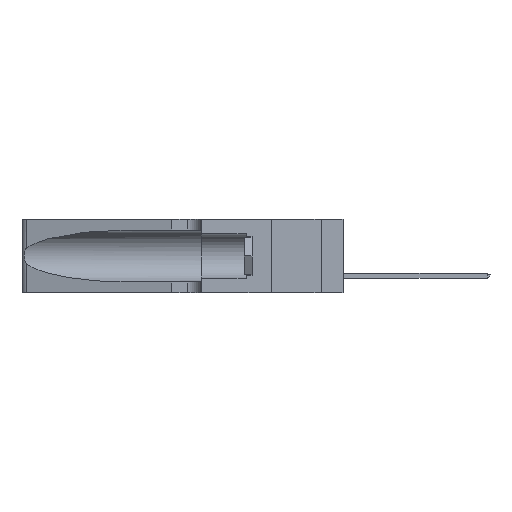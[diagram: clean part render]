
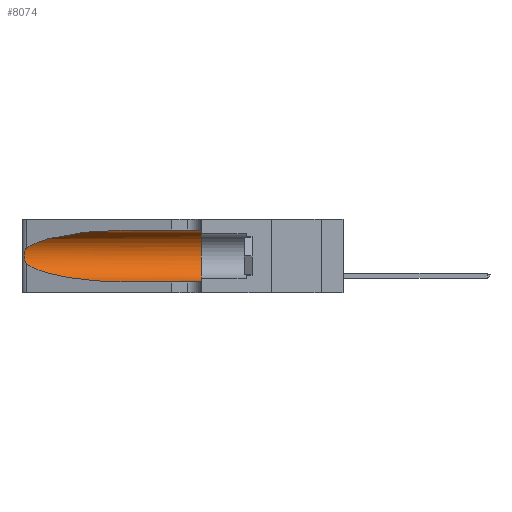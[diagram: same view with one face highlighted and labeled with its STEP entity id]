
A CAD part, left-side view. The second image highlights one B-rep face of the part: STEP entity #8074.
In plain terms, the highlighted cylindrical face has radius 3.308 mm (diameter 6.617 mm), a partial arc.
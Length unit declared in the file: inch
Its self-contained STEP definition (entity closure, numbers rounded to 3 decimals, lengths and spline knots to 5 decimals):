
#131 = EDGE_CURVE ( 'NONE', #30918, #43896, #28173, .T. ) ;
#206 = AXIS2_PLACEMENT_3D ( 'NONE', #17115, #22772, #15755 ) ;
#1031 = CARTESIAN_POINT ( 'NONE',  ( 0.1305, 0.35, 0.05475 ) ) ;
#1728 = B_SPLINE_CURVE_WITH_KNOTS ( 'NONE', 3,
 ( #28194, #2539, #35763, #24893, #32427, #6935, #26550, #5918, #18205, #4153, #21812, #35716, #33601, #24954 ),
 .UNSPECIFIED., .F., .F.,
 ( 4, 2, 2, 2, 2, 2, 4 ),
 ( 0., 0.00027, 0.00053, 0.00107, 0.0016, 0.00187, 0.00214 ),
 .UNSPECIFIED. ) ;
#2324 = DIRECTION ( 'NONE',  ( 0., 0., -1. ) ) ;
#2539 = CARTESIAN_POINT ( 'NONE',  ( 0.25555, 1.22994, 0.2215 ) ) ;
#4153 = CARTESIAN_POINT ( 'NONE',  ( 0.25856, 1.23593, 0.16098 ) ) ;
#4603 = CARTESIAN_POINT ( 'NONE',  ( 0.25487, 1.22718, 0.22369 ) ) ;
#4626 =( BOUNDED_CURVE ( )  B_SPLINE_CURVE ( 3, ( #16541, #5074, #40308, #4603 ),
 .UNSPECIFIED., .F., .F. ) 
 B_SPLINE_CURVE_WITH_KNOTS ( ( 4, 4 ),
 ( 1.5708, 2.84003 ),
 .UNSPECIFIED. ) 
 CURVE ( )  GEOMETRIC_REPRESENTATION_ITEM ( )  RATIONAL_B_SPLINE_CURVE ( ( 1., 0.87, 0.87, 1. ) ) 
 REPRESENTATION_ITEM ( '' )  );
#4814 = DIRECTION ( 'NONE',  ( 0., -1., 0. ) ) ;
#4993 = CARTESIAN_POINT ( 'NONE',  ( 0.1305, 1.61858, 0.185 ) ) ;
#5074 = CARTESIAN_POINT ( 'NONE',  ( 0.18966, 0.96281, 0.31525 ) ) ;
#5448 = VERTEX_POINT ( 'NONE', #12905 ) ;
#5918 = CARTESIAN_POINT ( 'NONE',  ( 0.26075, 1.23896, 0.178 ) ) ;
#6399 = AXIS2_PLACEMENT_3D ( 'NONE', #4993, #19834, #2324 ) ;
#6935 = CARTESIAN_POINT ( 'NONE',  ( 0.26018, 1.23835, 0.19895 ) ) ;
#7146 = VERTEX_POINT ( 'NONE', #20225 ) ;
#7177 = CARTESIAN_POINT ( 'NONE',  ( 0.1305, 0.72297, 0.05475 ) ) ;
#7423 = CARTESIAN_POINT ( 'NONE',  ( 0.1305, 0.72297, 0.05475 ) ) ;
#8074 = ADVANCED_FACE ( 'NONE', ( #23088 ), #19157, .F. ) ;
#8538 = ORIENTED_EDGE ( 'NONE', *, *, #16496, .T. ) ;
#8761 = CARTESIAN_POINT ( 'NONE',  ( 0.1305, 1.61858, 0.05475 ) ) ;
#9123 = ORIENTED_EDGE ( 'NONE', *, *, #36473, .F. ) ;
#9232 = LINE ( 'NONE', #22787, #46150 ) ;
#11258 = EDGE_CURVE ( 'NONE', #43896, #36379, #15746, .T. ) ;
#12360 = EDGE_CURVE ( 'NONE', #5448, #30918, #1728, .T. ) ;
#12905 = CARTESIAN_POINT ( 'NONE',  ( 0.25487, 1.22718, 0.22369 ) ) ;
#13429 = EDGE_CURVE ( 'NONE', #15720, #36379, #40744, .T. ) ;
#15720 = VERTEX_POINT ( 'NONE', #25858 ) ;
#15746 = LINE ( 'NONE', #8761, #39845 ) ;
#15755 = DIRECTION ( 'NONE',  ( 0., 0., 1. ) ) ;
#16496 = EDGE_CURVE ( 'NONE', #7146, #5448, #4626, .T. ) ;
#16541 = CARTESIAN_POINT ( 'NONE',  ( 0.1305, 0.72297, 0.31525 ) ) ;
#17115 = CARTESIAN_POINT ( 'NONE',  ( 0.1305, 0.35, 0.185 ) ) ;
#18205 = CARTESIAN_POINT ( 'NONE',  ( 0.26017, 1.23833, 0.17102 ) ) ;
#19157 = CYLINDRICAL_SURFACE ( 'NONE', #6399, 0.13025 ) ;
#19531 = ORIENTED_EDGE ( 'NONE', *, *, #11258, .T. ) ;
#19834 = DIRECTION ( 'NONE',  ( 0., -1., 0. ) ) ;
#20225 = CARTESIAN_POINT ( 'NONE',  ( 0.1305, 0.72297, 0.31525 ) ) ;
#21625 = CARTESIAN_POINT ( 'NONE',  ( 0.2373, 1.15595, 0.08982 ) ) ;
#21812 = CARTESIAN_POINT ( 'NONE',  ( 0.25789, 1.23486, 0.15765 ) ) ;
#22772 = DIRECTION ( 'NONE',  ( 0., 1., 0. ) ) ;
#22787 = CARTESIAN_POINT ( 'NONE',  ( 0.1305, 1.61858, 0.31525 ) ) ;
#23088 = FACE_OUTER_BOUND ( 'NONE', #45938, .T. ) ;
#24893 = CARTESIAN_POINT ( 'NONE',  ( 0.25787, 1.23484, 0.2124 ) ) ;
#24954 = CARTESIAN_POINT ( 'NONE',  ( 0.25487, 1.22718, 0.14631 ) ) ;
#25858 = CARTESIAN_POINT ( 'NONE',  ( 0.1305, 0.35, 0.31525 ) ) ;
#26370 = ORIENTED_EDGE ( 'NONE', *, *, #12360, .T. ) ;
#26550 = CARTESIAN_POINT ( 'NONE',  ( 0.26075, 1.23896, 0.19203 ) ) ;
#28173 =( BOUNDED_CURVE ( )  B_SPLINE_CURVE ( 3, ( #35824, #21625, #28858, #7423 ),
 .UNSPECIFIED., .F., .F. ) 
 B_SPLINE_CURVE_WITH_KNOTS ( ( 4, 4 ),
 ( 3.44316, 4.71239 ),
 .UNSPECIFIED. ) 
 CURVE ( )  GEOMETRIC_REPRESENTATION_ITEM ( )  RATIONAL_B_SPLINE_CURVE ( ( 1., 0.87, 0.87, 1. ) ) 
 REPRESENTATION_ITEM ( '' )  );
#28194 = CARTESIAN_POINT ( 'NONE',  ( 0.25487, 1.22718, 0.22369 ) ) ;
#28858 = CARTESIAN_POINT ( 'NONE',  ( 0.18966, 0.96281, 0.05475 ) ) ;
#30918 = VERTEX_POINT ( 'NONE', #40279 ) ;
#32427 = CARTESIAN_POINT ( 'NONE',  ( 0.25854, 1.2359, 0.20912 ) ) ;
#33601 = CARTESIAN_POINT ( 'NONE',  ( 0.25555, 1.22993, 0.14849 ) ) ;
#35716 = CARTESIAN_POINT ( 'NONE',  ( 0.25639, 1.23186, 0.15144 ) ) ;
#35763 = CARTESIAN_POINT ( 'NONE',  ( 0.25639, 1.23184, 0.21858 ) ) ;
#35824 = CARTESIAN_POINT ( 'NONE',  ( 0.25487, 1.22718, 0.14631 ) ) ;
#36379 = VERTEX_POINT ( 'NONE', #1031 ) ;
#36473 = EDGE_CURVE ( 'NONE', #7146, #15720, #9232, .T. ) ;
#38036 = ORIENTED_EDGE ( 'NONE', *, *, #131, .T. ) ;
#39845 = VECTOR ( 'NONE', #44893, 39.37008 ) ;
#40279 = CARTESIAN_POINT ( 'NONE',  ( 0.25487, 1.22718, 0.14631 ) ) ;
#40308 = CARTESIAN_POINT ( 'NONE',  ( 0.2373, 1.15595, 0.28018 ) ) ;
#40744 = CIRCLE ( 'NONE', #206, 0.13025 ) ;
#42663 = ORIENTED_EDGE ( 'NONE', *, *, #13429, .F. ) ;
#43896 = VERTEX_POINT ( 'NONE', #7177 ) ;
#44893 = DIRECTION ( 'NONE',  ( 0., -1., 0. ) ) ;
#45938 = EDGE_LOOP ( 'NONE', ( #8538, #26370, #38036, #19531, #42663, #9123 ) ) ;
#46150 = VECTOR ( 'NONE', #4814, 39.37008 ) ;
